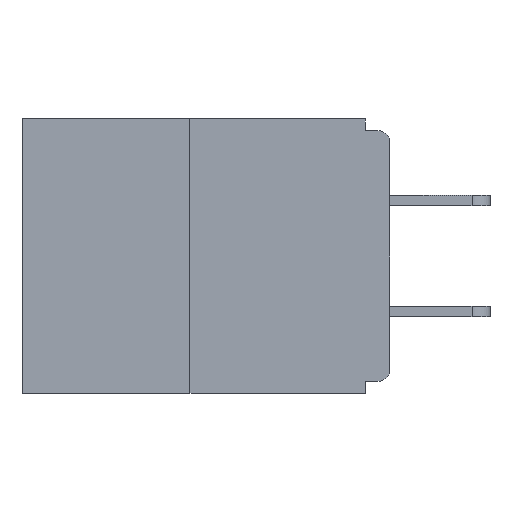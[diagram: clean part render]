
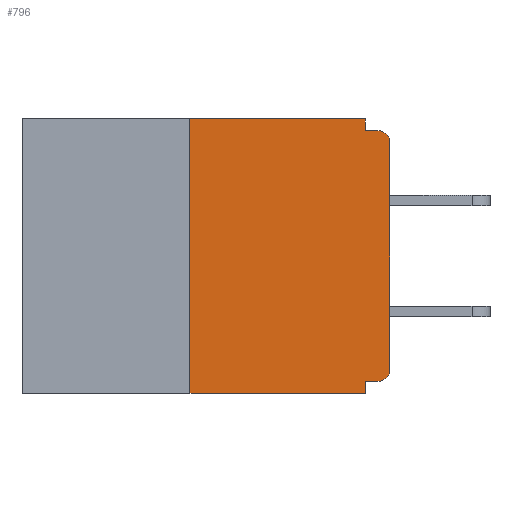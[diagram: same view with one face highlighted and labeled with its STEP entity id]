
A CAD part, left-side view. The second image highlights one B-rep face of the part: STEP entity #796.
In plain terms, the highlighted planar face has unit normal (-1, 0, 0).
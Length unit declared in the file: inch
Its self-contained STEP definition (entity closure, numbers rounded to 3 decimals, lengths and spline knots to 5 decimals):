
#184 = VERTEX_POINT ( 'NONE', #6891 ) ;
#426 = DIRECTION ( 'NONE',  ( 0., 0., -1. ) ) ;
#522 = CIRCLE ( 'NONE', #11658, 0.015 ) ;
#740 = FACE_OUTER_BOUND ( 'NONE', #798, .T. ) ;
#781 = VERTEX_POINT ( 'NONE', #9855 ) ;
#796 = ADVANCED_FACE ( 'NONE', ( #740 ), #5583, .F. ) ;
#798 = EDGE_LOOP ( 'NONE', ( #5300, #5776, #5055, #964, #9143, #4357, #5239, #1530, #10331, #9795 ) ) ;
#855 = CARTESIAN_POINT ( 'NONE',  ( 0., 0.015, -0.313 ) ) ;
#964 = ORIENTED_EDGE ( 'NONE', *, *, #12870, .F. ) ;
#1041 = VECTOR ( 'NONE', #3270, 39.37008 ) ;
#1530 = ORIENTED_EDGE ( 'NONE', *, *, #7389, .T. ) ;
#2180 = LINE ( 'NONE', #6182, #7047 ) ;
#2205 = EDGE_CURVE ( 'NONE', #184, #6351, #12713, .T. ) ;
#2329 = EDGE_CURVE ( 'NONE', #6351, #6291, #2180, .T. ) ;
#2418 = VECTOR ( 'NONE', #8204, 39.37008 ) ;
#2479 = DIRECTION ( 'NONE',  ( 1., 0., 0. ) ) ;
#2536 = CARTESIAN_POINT ( 'NONE',  ( 0., 0., 0. ) ) ;
#2641 = VERTEX_POINT ( 'NONE', #12085 ) ;
#2852 = DIRECTION ( 'NONE',  ( 0., 0., -1. ) ) ;
#2889 = CARTESIAN_POINT ( 'NONE',  ( 0., 0.031, -0.343 ) ) ;
#3126 = VECTOR ( 'NONE', #8700, 39.37008 ) ;
#3270 = DIRECTION ( 'NONE',  ( 0., -1., 0. ) ) ;
#3317 = CARTESIAN_POINT ( 'NONE',  ( 0., 0.015, -0.015 ) ) ;
#3499 = VECTOR ( 'NONE', #3579, 39.37008 ) ;
#3579 = DIRECTION ( 'NONE',  ( 0., 0., -1. ) ) ;
#4222 = LINE ( 'NONE', #2536, #13074 ) ;
#4357 = ORIENTED_EDGE ( 'NONE', *, *, #7616, .T. ) ;
#4957 = VECTOR ( 'NONE', #7612, 39.37008 ) ;
#4979 = CIRCLE ( 'NONE', #9952, 0.015 ) ;
#5021 = CARTESIAN_POINT ( 'NONE',  ( 0., 0.25, 0. ) ) ;
#5055 = ORIENTED_EDGE ( 'NONE', *, *, #9874, .T. ) ;
#5166 = DIRECTION ( 'NONE',  ( -1., 0., 0. ) ) ;
#5239 = ORIENTED_EDGE ( 'NONE', *, *, #10456, .T. ) ;
#5300 = ORIENTED_EDGE ( 'NONE', *, *, #8597, .F. ) ;
#5583 = PLANE ( 'NONE',  #6781 ) ;
#5776 = ORIENTED_EDGE ( 'NONE', *, *, #7956, .F. ) ;
#5962 = CARTESIAN_POINT ( 'NONE',  ( 0., 0.031, 0. ) ) ;
#6182 = CARTESIAN_POINT ( 'NONE',  ( 0., 0., -0.015 ) ) ;
#6291 = VERTEX_POINT ( 'NONE', #3317 ) ;
#6351 = VERTEX_POINT ( 'NONE', #13639 ) ;
#6555 = EDGE_CURVE ( 'NONE', #6759, #781, #8422, .T. ) ;
#6691 = CARTESIAN_POINT ( 'NONE',  ( 0., 0.46, 0. ) ) ;
#6759 = VERTEX_POINT ( 'NONE', #7640 ) ;
#6781 = AXIS2_PLACEMENT_3D ( 'NONE', #9817, #2479, #10976 ) ;
#6891 = CARTESIAN_POINT ( 'NONE',  ( 0., 0.031, 0. ) ) ;
#7047 = VECTOR ( 'NONE', #9466, 39.37008 ) ;
#7389 = EDGE_CURVE ( 'NONE', #9943, #6291, #522, .T. ) ;
#7612 = DIRECTION ( 'NONE',  ( 0., -1., 0. ) ) ;
#7616 = EDGE_CURVE ( 'NONE', #6759, #2641, #4979, .T. ) ;
#7640 = CARTESIAN_POINT ( 'NONE',  ( 0., 0.015, -0.328 ) ) ;
#7778 = LINE ( 'NONE', #6691, #4957 ) ;
#7956 = EDGE_CURVE ( 'NONE', #9636, #9263, #9969, .T. ) ;
#8035 = DIRECTION ( 'NONE',  ( 0., 0., 1. ) ) ;
#8204 = DIRECTION ( 'NONE',  ( 0., 1., 0. ) ) ;
#8422 = LINE ( 'NONE', #12639, #2418 ) ;
#8597 = EDGE_CURVE ( 'NONE', #9263, #184, #7778, .T. ) ;
#8700 = DIRECTION ( 'NONE',  ( 0., 0., 1. ) ) ;
#8728 = CARTESIAN_POINT ( 'NONE',  ( 0., 0.46, -0.343 ) ) ;
#8892 = DIRECTION ( 'NONE',  ( -1., 0., 0. ) ) ;
#9143 = ORIENTED_EDGE ( 'NONE', *, *, #6555, .F. ) ;
#9204 = CARTESIAN_POINT ( 'NONE',  ( 0., 0.25, -0.343 ) ) ;
#9263 = VERTEX_POINT ( 'NONE', #5021 ) ;
#9466 = DIRECTION ( 'NONE',  ( 0., -1., 0. ) ) ;
#9636 = VERTEX_POINT ( 'NONE', #9204 ) ;
#9795 = ORIENTED_EDGE ( 'NONE', *, *, #2205, .F. ) ;
#9817 = CARTESIAN_POINT ( 'NONE',  ( 0., 0.46, 0. ) ) ;
#9855 = CARTESIAN_POINT ( 'NONE',  ( 0., 0.031, -0.328 ) ) ;
#9874 = EDGE_CURVE ( 'NONE', #9636, #13767, #10075, .T. ) ;
#9943 = VERTEX_POINT ( 'NONE', #13115 ) ;
#9952 = AXIS2_PLACEMENT_3D ( 'NONE', #855, #5166, #11555 ) ;
#9969 = LINE ( 'NONE', #12020, #3126 ) ;
#10075 = LINE ( 'NONE', #8728, #1041 ) ;
#10331 = ORIENTED_EDGE ( 'NONE', *, *, #2329, .F. ) ;
#10456 = EDGE_CURVE ( 'NONE', #2641, #9943, #4222, .T. ) ;
#10976 = DIRECTION ( 'NONE',  ( 0., 0., -1. ) ) ;
#10989 = CARTESIAN_POINT ( 'NONE',  ( 0., 0.015, -0.03 ) ) ;
#11555 = DIRECTION ( 'NONE',  ( 0., 0., -1. ) ) ;
#11658 = AXIS2_PLACEMENT_3D ( 'NONE', #10989, #8892, #426 ) ;
#12020 = CARTESIAN_POINT ( 'NONE',  ( 0., 0.25, 0. ) ) ;
#12030 = LINE ( 'NONE', #12118, #3499 ) ;
#12085 = CARTESIAN_POINT ( 'NONE',  ( 0., 0., -0.313 ) ) ;
#12118 = CARTESIAN_POINT ( 'NONE',  ( 0., 0.031, -0.343 ) ) ;
#12639 = CARTESIAN_POINT ( 'NONE',  ( 0., 0., -0.328 ) ) ;
#12713 = LINE ( 'NONE', #5962, #13226 ) ;
#12870 = EDGE_CURVE ( 'NONE', #781, #13767, #12030, .T. ) ;
#13074 = VECTOR ( 'NONE', #8035, 39.37008 ) ;
#13115 = CARTESIAN_POINT ( 'NONE',  ( 0., 0., -0.03 ) ) ;
#13226 = VECTOR ( 'NONE', #2852, 39.37008 ) ;
#13639 = CARTESIAN_POINT ( 'NONE',  ( 0., 0.031, -0.015 ) ) ;
#13767 = VERTEX_POINT ( 'NONE', #2889 ) ;
